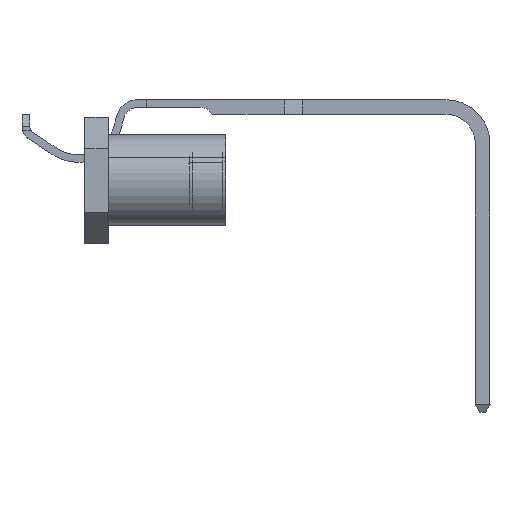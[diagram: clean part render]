
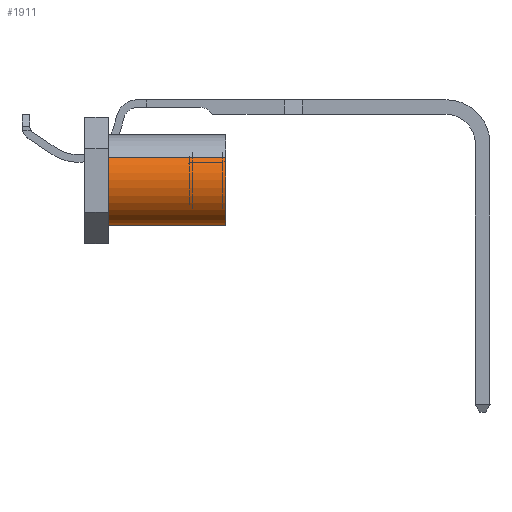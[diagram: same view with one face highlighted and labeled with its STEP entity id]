
A CAD part, left-side view. The second image highlights one B-rep face of the part: STEP entity #1911.
In plain terms, the highlighted cylindrical face has radius 1.968 mm (diameter 3.937 mm), a partial arc.
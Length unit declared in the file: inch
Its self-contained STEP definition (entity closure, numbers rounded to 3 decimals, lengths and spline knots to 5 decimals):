
#1911 = ADVANCED_FACE ( 'NONE', ( #13178 ), #17629, .T. ) ;
#2345 = ORIENTED_EDGE ( 'NONE', *, *, #15991, .F. ) ;
#2985 = EDGE_CURVE ( 'NONE', #4894, #18636, #15820, .T. ) ;
#4527 = CARTESIAN_POINT ( 'NONE',  ( 0., 0.24, 0.0775 ) ) ;
#4696 = ORIENTED_EDGE ( 'NONE', *, *, #12516, .F. ) ;
#4894 = VERTEX_POINT ( 'NONE', #11363 ) ;
#5717 = LINE ( 'NONE', #24006, #15362 ) ;
#5941 = DIRECTION ( 'NONE',  ( 0., 1., 0. ) ) ;
#6448 = EDGE_CURVE ( 'NONE', #18247, #4894, #5717, .T. ) ;
#6469 = ORIENTED_EDGE ( 'NONE', *, *, #6448, .T. ) ;
#6854 = DIRECTION ( 'NONE',  ( 0., -1., 0. ) ) ;
#8597 = EDGE_LOOP ( 'NONE', ( #4696, #2345, #6469, #17450 ) ) ;
#9758 = DIRECTION ( 'NONE',  ( 0., -1., 0. ) ) ;
#10531 = DIRECTION ( 'NONE',  ( 0., 1., 0. ) ) ;
#10735 = DIRECTION ( 'NONE',  ( 0., 0., -1. ) ) ;
#11363 = CARTESIAN_POINT ( 'NONE',  ( 0., 0.04, -0.0775 ) ) ;
#11705 = VECTOR ( 'NONE', #9758, 39.37008 ) ;
#12022 = AXIS2_PLACEMENT_3D ( 'NONE', #17410, #5941, #19308 ) ;
#12516 = EDGE_CURVE ( 'NONE', #17225, #18636, #16836, .T. ) ;
#13178 = FACE_OUTER_BOUND ( 'NONE', #8597, .T. ) ;
#14617 = CIRCLE ( 'NONE', #20347, 0.0775 ) ;
#14678 = DIRECTION ( 'NONE',  ( 0., -1., 0. ) ) ;
#15362 = VECTOR ( 'NONE', #6854, 39.37008 ) ;
#15820 = CIRCLE ( 'NONE', #12022, 0.0775 ) ;
#15991 = EDGE_CURVE ( 'NONE', #18247, #17225, #14617, .T. ) ;
#16836 = LINE ( 'NONE', #21232, #11705 ) ;
#16996 = AXIS2_PLACEMENT_3D ( 'NONE', #24152, #14678, #10735 ) ;
#17225 = VERTEX_POINT ( 'NONE', #4527 ) ;
#17410 = CARTESIAN_POINT ( 'NONE',  ( 0., 0.04, 0. ) ) ;
#17450 = ORIENTED_EDGE ( 'NONE', *, *, #2985, .T. ) ;
#17629 = CYLINDRICAL_SURFACE ( 'NONE', #16996, 0.0775 ) ;
#18247 = VERTEX_POINT ( 'NONE', #20162 ) ;
#18636 = VERTEX_POINT ( 'NONE', #19408 ) ;
#19308 = DIRECTION ( 'NONE',  ( 0., 0., 1. ) ) ;
#19408 = CARTESIAN_POINT ( 'NONE',  ( 0., 0.04, 0.0775 ) ) ;
#20162 = CARTESIAN_POINT ( 'NONE',  ( 0., 0.24, -0.0775 ) ) ;
#20347 = AXIS2_PLACEMENT_3D ( 'NONE', #22005, #10531, #23950 ) ;
#21232 = CARTESIAN_POINT ( 'NONE',  ( 0., 0.24, 0.0775 ) ) ;
#22005 = CARTESIAN_POINT ( 'NONE',  ( 0., 0.24, 0. ) ) ;
#23950 = DIRECTION ( 'NONE',  ( 0., 0., 1. ) ) ;
#24006 = CARTESIAN_POINT ( 'NONE',  ( 0., 0.24, -0.0775 ) ) ;
#24152 = CARTESIAN_POINT ( 'NONE',  ( 0., 0.24, 0. ) ) ;
